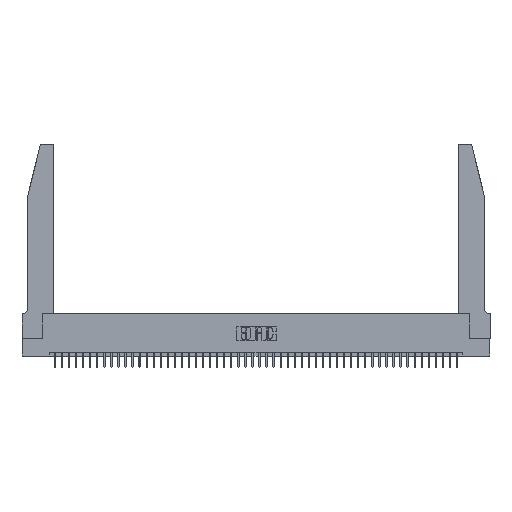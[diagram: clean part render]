
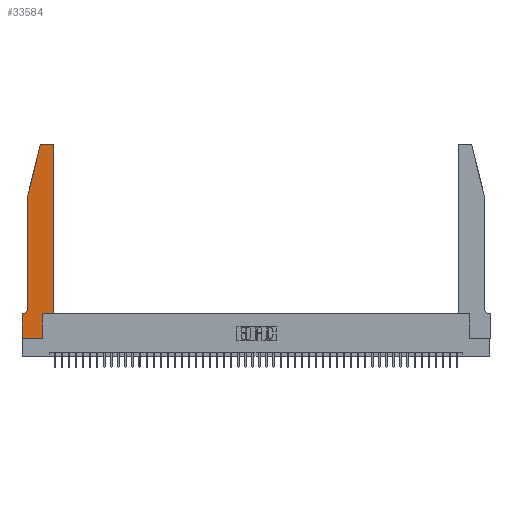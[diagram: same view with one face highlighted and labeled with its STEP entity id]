
A CAD part, top view. The second image highlights one B-rep face of the part: STEP entity #33584.
In plain terms, the highlighted planar face has unit normal (0, 0, 1).
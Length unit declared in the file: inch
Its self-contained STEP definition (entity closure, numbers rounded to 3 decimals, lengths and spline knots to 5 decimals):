
#748 = CARTESIAN_POINT ( 'NONE',  ( 0.4505, 2.72, 0.37 ) ) ;
#1658 = LINE ( 'NONE', #8393, #23129 ) ;
#1774 = CARTESIAN_POINT ( 'NONE',  ( 0.284, 2.75, 0.37 ) ) ;
#2538 = DIRECTION ( 'NONE',  ( 0., 0., 1. ) ) ;
#3535 = CARTESIAN_POINT ( 'NONE',  ( 0.0755, 2., 0.37 ) ) ;
#4567 = VERTEX_POINT ( 'NONE', #36159 ) ;
#5531 = VECTOR ( 'NONE', #46074, 39.37008 ) ;
#5594 = EDGE_CURVE ( 'NONE', #4567, #31563, #32542, .T. ) ;
#5601 = CARTESIAN_POINT ( 'NONE',  ( 0.4505, 0.35, 0.37 ) ) ;
#5733 = VECTOR ( 'NONE', #35222, 39.37008 ) ;
#6699 = CARTESIAN_POINT ( 'NONE',  ( 0.0755, 0.35, 0.37 ) ) ;
#6828 = ORIENTED_EDGE ( 'NONE', *, *, #5594, .T. ) ;
#7301 = CARTESIAN_POINT ( 'NONE',  ( 0.0055, 0.42, 0.37 ) ) ;
#8393 = CARTESIAN_POINT ( 'NONE',  ( 0.2605, 2.75, 0.37 ) ) ;
#9300 = VECTOR ( 'NONE', #25749, 39.37008 ) ;
#9554 = CIRCLE ( 'NONE', #18109, 0.07 ) ;
#9616 = CARTESIAN_POINT ( 'NONE',  ( 0.2865, 0., 0.37 ) ) ;
#10821 = ORIENTED_EDGE ( 'NONE', *, *, #25269, .T. ) ;
#11011 = EDGE_CURVE ( 'NONE', #35967, #29032, #32668, .T. ) ;
#11355 = LINE ( 'NONE', #5601, #5531 ) ;
#11858 = EDGE_CURVE ( 'NONE', #24047, #45909, #39543, .T. ) ;
#12572 = VECTOR ( 'NONE', #36724, 39.37008 ) ;
#12672 = CARTESIAN_POINT ( 'NONE',  ( 0.0755, 2., 0.37 ) ) ;
#12725 = VECTOR ( 'NONE', #24887, 39.37008 ) ;
#13302 = VECTOR ( 'NONE', #19284, 39.37008 ) ;
#13736 = CARTESIAN_POINT ( 'NONE',  ( 0.0755, 2., 0.37 ) ) ;
#14961 = ORIENTED_EDGE ( 'NONE', *, *, #47141, .T. ) ;
#15273 = EDGE_CURVE ( 'NONE', #15839, #18195, #9554, .T. ) ;
#15839 = VERTEX_POINT ( 'NONE', #36488 ) ;
#15843 = VERTEX_POINT ( 'NONE', #36977 ) ;
#15995 = ORIENTED_EDGE ( 'NONE', *, *, #44260, .T. ) ;
#16779 = EDGE_CURVE ( 'NONE', #29032, #40848, #43743, .T. ) ;
#18109 = AXIS2_PLACEMENT_3D ( 'NONE', #7301, #33283, #18513 ) ;
#18195 = VERTEX_POINT ( 'NONE', #41465 ) ;
#18513 = DIRECTION ( 'NONE',  ( -1., 0., 0. ) ) ;
#18742 = CARTESIAN_POINT ( 'NONE',  ( 0., 0., 0.37 ) ) ;
#18768 = EDGE_CURVE ( 'NONE', #40848, #15839, #36562, .T. ) ;
#19001 = EDGE_CURVE ( 'NONE', #31563, #15843, #30713, .T. ) ;
#19108 = DIRECTION ( 'NONE',  ( 1., 0., 0. ) ) ;
#19136 = DIRECTION ( 'NONE',  ( -1., 0., 0. ) ) ;
#19284 = DIRECTION ( 'NONE',  ( 0., -1., 0. ) ) ;
#19546 = ORIENTED_EDGE ( 'NONE', *, *, #28300, .T. ) ;
#19559 = VERTEX_POINT ( 'NONE', #46867 ) ;
#20046 = CARTESIAN_POINT ( 'NONE',  ( 0.4205, 2.72, 0.37 ) ) ;
#20386 = CARTESIAN_POINT ( 'NONE',  ( 0.2865, 0.35, 0.37 ) ) ;
#22287 = ORIENTED_EDGE ( 'NONE', *, *, #15273, .T. ) ;
#22950 = CARTESIAN_POINT ( 'NONE',  ( 0.25487, 2.72718, 0.37 ) ) ;
#23129 = VECTOR ( 'NONE', #19136, 39.37008 ) ;
#23332 = AXIS2_PLACEMENT_3D ( 'NONE', #36158, #39749, #24790 ) ;
#24047 = VERTEX_POINT ( 'NONE', #748 ) ;
#24275 = DIRECTION ( 'NONE',  ( 1., 0., 0. ) ) ;
#24790 = DIRECTION ( 'NONE',  ( 1., 0., 0. ) ) ;
#24805 = CARTESIAN_POINT ( 'NONE',  ( 0.284, 2.72, 0.37 ) ) ;
#24887 = DIRECTION ( 'NONE',  ( -1., 0., 0. ) ) ;
#25269 = EDGE_CURVE ( 'NONE', #18195, #19559, #30140, .T. ) ;
#25567 = ORIENTED_EDGE ( 'NONE', *, *, #11858, .T. ) ;
#25749 = DIRECTION ( 'NONE',  ( 0., -1., 0. ) ) ;
#26969 = VERTEX_POINT ( 'NONE', #40565 ) ;
#27098 = ORIENTED_EDGE ( 'NONE', *, *, #16779, .T. ) ;
#27530 = DIRECTION ( 'NONE',  ( 0., 0., 1. ) ) ;
#27878 = VECTOR ( 'NONE', #19108, 39.37008 ) ;
#28300 = EDGE_CURVE ( 'NONE', #45909, #35967, #1658, .T. ) ;
#28519 = DIRECTION ( 'NONE',  ( 1., 0., 0. ) ) ;
#28838 = PLANE ( 'NONE',  #23332 ) ;
#29032 = VERTEX_POINT ( 'NONE', #22950 ) ;
#29426 = CARTESIAN_POINT ( 'NONE',  ( 0.4205, 2.75, 0.37 ) ) ;
#30140 = LINE ( 'NONE', #6699, #12725 ) ;
#30687 = AXIS2_PLACEMENT_3D ( 'NONE', #24805, #2538, #28519 ) ;
#30713 = LINE ( 'NONE', #20386, #5733 ) ;
#31563 = VERTEX_POINT ( 'NONE', #9616 ) ;
#32542 = LINE ( 'NONE', #34550, #27878 ) ;
#32668 = CIRCLE ( 'NONE', #30687, 0.03 ) ;
#33283 = DIRECTION ( 'NONE',  ( 0., 0., -1. ) ) ;
#33584 = ADVANCED_FACE ( 'NONE', ( #42712 ), #28838, .T. ) ;
#33861 = VECTOR ( 'NONE', #38675, 39.37008 ) ;
#34550 = CARTESIAN_POINT ( 'NONE',  ( 0., 0., 0.37 ) ) ;
#35222 = DIRECTION ( 'NONE',  ( 0., 1., 0. ) ) ;
#35850 = LINE ( 'NONE', #43555, #12572 ) ;
#35967 = VERTEX_POINT ( 'NONE', #1774 ) ;
#36158 = CARTESIAN_POINT ( 'NONE',  ( 0., 0.35, 0.37 ) ) ;
#36159 = CARTESIAN_POINT ( 'NONE',  ( 0., 0., 0.37 ) ) ;
#36488 = CARTESIAN_POINT ( 'NONE',  ( 0.0755, 0.42, 0.37 ) ) ;
#36562 = LINE ( 'NONE', #3535, #13302 ) ;
#36724 = DIRECTION ( 'NONE',  ( 0., 1., 0. ) ) ;
#36977 = CARTESIAN_POINT ( 'NONE',  ( 0.2865, 0.35, 0.37 ) ) ;
#37185 = ORIENTED_EDGE ( 'NONE', *, *, #11011, .T. ) ;
#38302 = EDGE_CURVE ( 'NONE', #26969, #24047, #35850, .T. ) ;
#38675 = DIRECTION ( 'NONE',  ( -0.239, -0.971, 0. ) ) ;
#39543 = CIRCLE ( 'NONE', #46018, 0.03 ) ;
#39749 = DIRECTION ( 'NONE',  ( 0., 0., 1. ) ) ;
#40565 = CARTESIAN_POINT ( 'NONE',  ( 0.4505, 0.35, 0.37 ) ) ;
#40848 = VERTEX_POINT ( 'NONE', #13736 ) ;
#41327 = EDGE_LOOP ( 'NONE', ( #19546, #37185, #27098, #47093, #22287, #10821, #14961, #6828, #46689, #15995, #41957, #25567 ) ) ;
#41465 = CARTESIAN_POINT ( 'NONE',  ( 0.0055, 0.35, 0.37 ) ) ;
#41957 = ORIENTED_EDGE ( 'NONE', *, *, #38302, .T. ) ;
#42712 = FACE_OUTER_BOUND ( 'NONE', #41327, .T. ) ;
#43555 = CARTESIAN_POINT ( 'NONE',  ( 0.4505, 0.35, 0.37 ) ) ;
#43743 = LINE ( 'NONE', #12672, #33861 ) ;
#44192 = LINE ( 'NONE', #18742, #9300 ) ;
#44260 = EDGE_CURVE ( 'NONE', #15843, #26969, #11355, .T. ) ;
#45909 = VERTEX_POINT ( 'NONE', #29426 ) ;
#46018 = AXIS2_PLACEMENT_3D ( 'NONE', #20046, #27530, #24275 ) ;
#46074 = DIRECTION ( 'NONE',  ( 1., 0., 0. ) ) ;
#46689 = ORIENTED_EDGE ( 'NONE', *, *, #19001, .T. ) ;
#46867 = CARTESIAN_POINT ( 'NONE',  ( 0., 0.35, 0.37 ) ) ;
#47093 = ORIENTED_EDGE ( 'NONE', *, *, #18768, .T. ) ;
#47141 = EDGE_CURVE ( 'NONE', #19559, #4567, #44192, .T. ) ;
